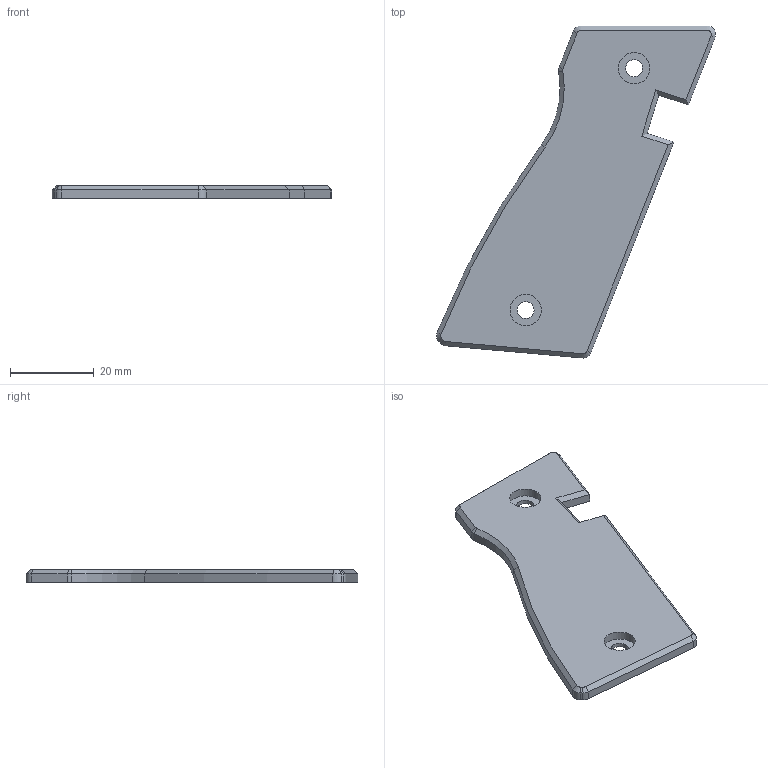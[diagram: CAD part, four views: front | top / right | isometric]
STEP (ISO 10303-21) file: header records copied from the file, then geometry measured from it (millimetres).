
FILE_DESCRIPTION(/* description */ (''),/* implementation_level */ '2;1');
FILE_NAME(/* name */ 'G19Eleven Right Flat Grip.step',/* time_stamp */ '2022-05-10T10:24:07-06:00',/* author */ (''),/* organization */ (''),/* preprocessor_version */ 'ST-DEVELOPER v18.1',/* originating_system */ 'Autodesk Translation Framework v10.14.0.1471',/* authorisation */ '');
FILE_SCHEMA (('AUTOMOTIVE_DESIGN { 1 0 10303 214 3 1 1 }'));
Length unit declared in the file: millimetre
Products named in the file (1): G1911
Bounding box: 66.52 x 79.14 x 3 mm (x, y, z)
Volume: 7592.2 mm3; surface area: 5952.3 mm2
Topology: 1 solids, 1 shells, 42 faces, 97 edges, 59 vertices
Faces by surface type: plane 22, cylinder 12, cone 8
Full cylindrical faces by diameter (mm): 4 x2, 7.5 x2
Entity records: 1239 total; most frequent: DIRECTION 214, CARTESIAN_POINT 208, ORIENTED_EDGE 194, EDGE_CURVE 97, AXIS2_PLACEMENT_3D 75, LINE 64, VECTOR 64, VERTEX_POINT 59
